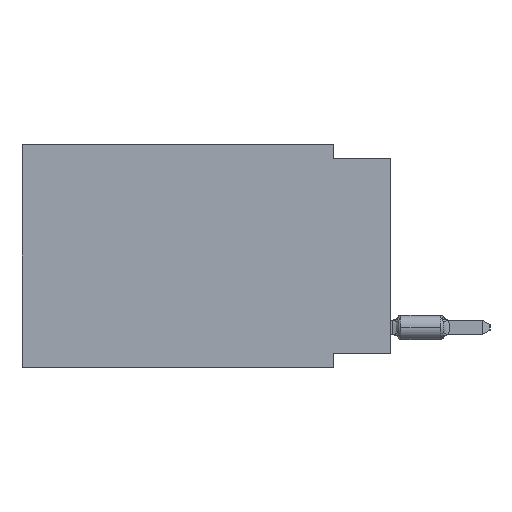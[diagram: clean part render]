
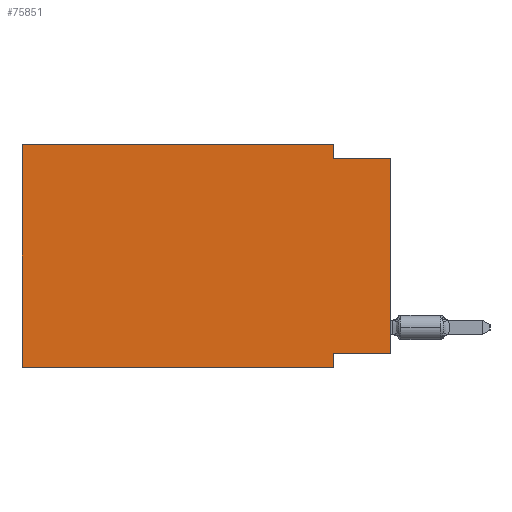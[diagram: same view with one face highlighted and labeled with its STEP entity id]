
A CAD part, left-side view. The second image highlights one B-rep face of the part: STEP entity #75851.
In plain terms, the highlighted planar face has unit normal (-1, 0, 0).
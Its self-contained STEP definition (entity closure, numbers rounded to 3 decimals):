
#1581 = AXIS2_PLACEMENT_3D ( 'NONE', #1866, #13999, #56813 ) ;
#1866 = CARTESIAN_POINT ( 'NONE',  ( 0., 16.383, 0. ) ) ;
#2692 = DIRECTION ( 'NONE',  ( 0., -1., 0. ) ) ;
#6042 = EDGE_CURVE ( 'NONE', #78683, #17483, #7222, .T. ) ;
#7222 = LINE ( 'NONE', #18546, #70080 ) ;
#8596 = LINE ( 'NONE', #15055, #25717 ) ;
#8773 = LINE ( 'NONE', #33421, #27505 ) ;
#9156 = DIRECTION ( 'NONE',  ( 0., 0., 1. ) ) ;
#9621 = DIRECTION ( 'NONE',  ( 0., -1., 0. ) ) ;
#10831 = CARTESIAN_POINT ( 'NONE',  ( 0., 16.383, 0. ) ) ;
#13603 = FACE_OUTER_BOUND ( 'NONE', #54719, .T. ) ;
#13999 = DIRECTION ( 'NONE',  ( 1., 0., 0. ) ) ;
#14893 = VERTEX_POINT ( 'NONE', #44668 ) ;
#15055 = CARTESIAN_POINT ( 'NONE',  ( 0., 2.54, -9.906 ) ) ;
#15866 = ORIENTED_EDGE ( 'NONE', *, *, #36642, .F. ) ;
#17002 = CARTESIAN_POINT ( 'NONE',  ( 0., 2.54, 0. ) ) ;
#17483 = VERTEX_POINT ( 'NONE', #28855 ) ;
#18546 = CARTESIAN_POINT ( 'NONE',  ( 0., 0., -9.271 ) ) ;
#21032 = CARTESIAN_POINT ( 'NONE',  ( 0., 2.54, -9.906 ) ) ;
#21286 = LINE ( 'NONE', #51980, #44317 ) ;
#24809 = VERTEX_POINT ( 'NONE', #61799 ) ;
#25717 = VECTOR ( 'NONE', #64327, 1000. ) ;
#27283 = CARTESIAN_POINT ( 'NONE',  ( 0., 0., -0.635 ) ) ;
#27505 = VECTOR ( 'NONE', #2692, 1000. ) ;
#28855 = CARTESIAN_POINT ( 'NONE',  ( 0., 2.54, -9.271 ) ) ;
#29376 = LINE ( 'NONE', #55607, #68591 ) ;
#32509 = EDGE_CURVE ( 'NONE', #17483, #66773, #8596, .T. ) ;
#33421 = CARTESIAN_POINT ( 'NONE',  ( 0., 0., -0.635 ) ) ;
#36642 = EDGE_CURVE ( 'NONE', #24809, #55613, #79226, .T. ) ;
#37465 = EDGE_CURVE ( 'NONE', #55613, #76130, #8773, .T. ) ;
#38243 = PLANE ( 'NONE',  #1581 ) ;
#39034 = VECTOR ( 'NONE', #67199, 1000. ) ;
#39383 = DIRECTION ( 'NONE',  ( 0., 0., -1. ) ) ;
#40316 = LINE ( 'NONE', #10831, #59644 ) ;
#41826 = CARTESIAN_POINT ( 'NONE',  ( 0., 0., -9.271 ) ) ;
#41878 = CARTESIAN_POINT ( 'NONE',  ( 0., 2.54, -0.635 ) ) ;
#42691 = DIRECTION ( 'NONE',  ( 0., -1., 0. ) ) ;
#43183 = DIRECTION ( 'NONE',  ( 0., 1., 0. ) ) ;
#44317 = VECTOR ( 'NONE', #9156, 1000. ) ;
#44668 = CARTESIAN_POINT ( 'NONE',  ( 0., 16.383, -9.906 ) ) ;
#47107 = ORIENTED_EDGE ( 'NONE', *, *, #69348, .T. ) ;
#49362 = VECTOR ( 'NONE', #39383, 1000. ) ;
#49653 = EDGE_CURVE ( 'NONE', #76709, #24809, #40316, .T. ) ;
#51980 = CARTESIAN_POINT ( 'NONE',  ( 0., 16.383, 0. ) ) ;
#54258 = EDGE_CURVE ( 'NONE', #14893, #76709, #21286, .T. ) ;
#54719 = EDGE_LOOP ( 'NONE', ( #47107, #57041, #15866, #75702, #65539, #73761, #60126, #57921 ) ) ;
#55607 = CARTESIAN_POINT ( 'NONE',  ( 0., 16.383, -9.906 ) ) ;
#55613 = VERTEX_POINT ( 'NONE', #41878 ) ;
#56813 = DIRECTION ( 'NONE',  ( 0., 0., -1. ) ) ;
#57041 = ORIENTED_EDGE ( 'NONE', *, *, #37465, .F. ) ;
#57921 = ORIENTED_EDGE ( 'NONE', *, *, #6042, .F. ) ;
#59644 = VECTOR ( 'NONE', #9621, 1000. ) ;
#60126 = ORIENTED_EDGE ( 'NONE', *, *, #32509, .F. ) ;
#61799 = CARTESIAN_POINT ( 'NONE',  ( 0., 2.54, 0. ) ) ;
#64327 = DIRECTION ( 'NONE',  ( 0., 0., -1. ) ) ;
#65539 = ORIENTED_EDGE ( 'NONE', *, *, #54258, .F. ) ;
#66396 = LINE ( 'NONE', #78521, #39034 ) ;
#66773 = VERTEX_POINT ( 'NONE', #21032 ) ;
#67199 = DIRECTION ( 'NONE',  ( 0., 0., 1. ) ) ;
#68591 = VECTOR ( 'NONE', #42691, 1000. ) ;
#69348 = EDGE_CURVE ( 'NONE', #78683, #76130, #66396, .T. ) ;
#70080 = VECTOR ( 'NONE', #43183, 1000. ) ;
#73761 = ORIENTED_EDGE ( 'NONE', *, *, #75760, .T. ) ;
#74286 = CARTESIAN_POINT ( 'NONE',  ( 0., 16.383, 0. ) ) ;
#75702 = ORIENTED_EDGE ( 'NONE', *, *, #49653, .F. ) ;
#75760 = EDGE_CURVE ( 'NONE', #14893, #66773, #29376, .T. ) ;
#75851 = ADVANCED_FACE ( 'NONE', ( #13603 ), #38243, .F. ) ;
#76130 = VERTEX_POINT ( 'NONE', #27283 ) ;
#76709 = VERTEX_POINT ( 'NONE', #74286 ) ;
#78521 = CARTESIAN_POINT ( 'NONE',  ( 0., 0., 0. ) ) ;
#78683 = VERTEX_POINT ( 'NONE', #41826 ) ;
#79226 = LINE ( 'NONE', #17002, #49362 ) ;
